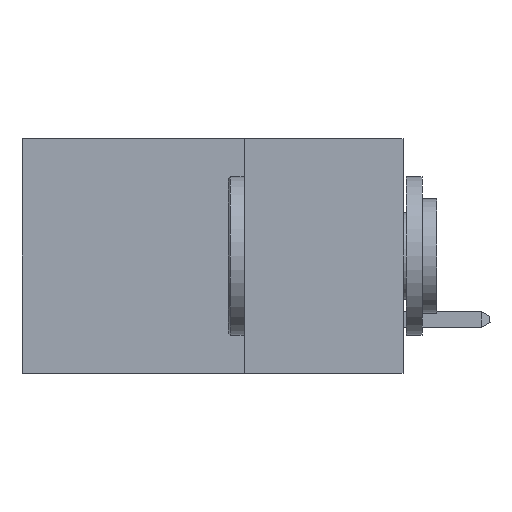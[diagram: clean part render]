
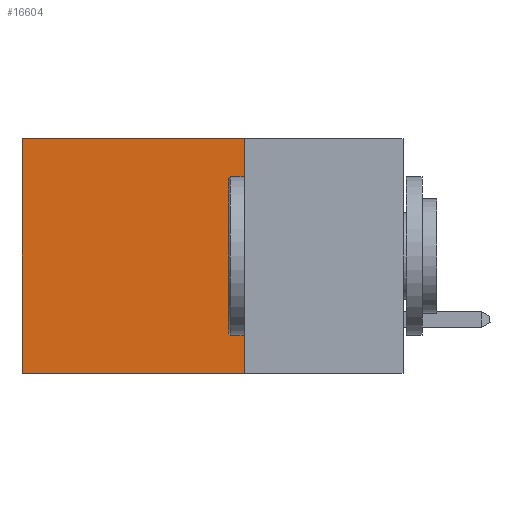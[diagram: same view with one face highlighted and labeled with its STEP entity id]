
A CAD part, left-side view. The second image highlights one B-rep face of the part: STEP entity #16604.
In plain terms, the highlighted planar face has unit normal (-1, 0, 0).
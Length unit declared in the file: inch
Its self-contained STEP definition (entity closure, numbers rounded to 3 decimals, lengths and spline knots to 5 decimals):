
#802 = VERTEX_POINT ( 'NONE', #10958 ) ;
#1083 = ORIENTED_EDGE ( 'NONE', *, *, #8094, .F. ) ;
#1933 = EDGE_CURVE ( 'NONE', #12147, #5858, #9127, .T. ) ;
#3163 = CARTESIAN_POINT ( 'NONE',  ( 0.2875, 0.25, 0. ) ) ;
#3304 = LINE ( 'NONE', #19776, #7354 ) ;
#3357 = DIRECTION ( 'NONE',  ( 0., 1., 0. ) ) ;
#3700 = LINE ( 'NONE', #11041, #11645 ) ;
#3724 = FACE_OUTER_BOUND ( 'NONE', #15707, .T. ) ;
#4468 = AXIS2_PLACEMENT_3D ( 'NONE', #17608, #19237, #9381 ) ;
#4553 = VECTOR ( 'NONE', #3357, 39.37008 ) ;
#5858 = VERTEX_POINT ( 'NONE', #17519 ) ;
#6473 = EDGE_CURVE ( 'NONE', #7257, #802, #3304, .T. ) ;
#7257 = VERTEX_POINT ( 'NONE', #9187 ) ;
#7354 = VECTOR ( 'NONE', #19843, 39.37008 ) ;
#8094 = EDGE_CURVE ( 'NONE', #12147, #7257, #3700, .T. ) ;
#9050 = DIRECTION ( 'NONE',  ( 0., 0., -1. ) ) ;
#9127 = LINE ( 'NONE', #3163, #4553 ) ;
#9187 = CARTESIAN_POINT ( 'NONE',  ( 0.2875, 0.25, -0.37 ) ) ;
#9381 = DIRECTION ( 'NONE',  ( 0., 0., -1. ) ) ;
#10724 = CARTESIAN_POINT ( 'NONE',  ( 0.2875, 0.6, 0. ) ) ;
#10958 = CARTESIAN_POINT ( 'NONE',  ( 0.2875, 0.6, -0.37 ) ) ;
#11041 = CARTESIAN_POINT ( 'NONE',  ( 0.2875, 0.25, 0. ) ) ;
#11085 = DIRECTION ( 'NONE',  ( 0., 0., -1. ) ) ;
#11195 = VECTOR ( 'NONE', #9050, 39.37008 ) ;
#11645 = VECTOR ( 'NONE', #11085, 39.37008 ) ;
#11924 = ORIENTED_EDGE ( 'NONE', *, *, #6473, .F. ) ;
#12147 = VERTEX_POINT ( 'NONE', #19243 ) ;
#15056 = LINE ( 'NONE', #10724, #11195 ) ;
#15707 = EDGE_LOOP ( 'NONE', ( #15827, #11924, #1083, #17468 ) ) ;
#15827 = ORIENTED_EDGE ( 'NONE', *, *, #15850, .T. ) ;
#15850 = EDGE_CURVE ( 'NONE', #5858, #802, #15056, .T. ) ;
#15971 = PLANE ( 'NONE',  #4468 ) ;
#16604 = ADVANCED_FACE ( 'NONE', ( #3724 ), #15971, .F. ) ;
#17468 = ORIENTED_EDGE ( 'NONE', *, *, #1933, .T. ) ;
#17519 = CARTESIAN_POINT ( 'NONE',  ( 0.2875, 0.6, 0. ) ) ;
#17608 = CARTESIAN_POINT ( 'NONE',  ( 0.2875, 0.25, 0. ) ) ;
#19237 = DIRECTION ( 'NONE',  ( 1., 0., 0. ) ) ;
#19243 = CARTESIAN_POINT ( 'NONE',  ( 0.2875, 0.25, 0. ) ) ;
#19776 = CARTESIAN_POINT ( 'NONE',  ( 0.2875, 0.25, -0.37 ) ) ;
#19843 = DIRECTION ( 'NONE',  ( 0., 1., 0. ) ) ;
